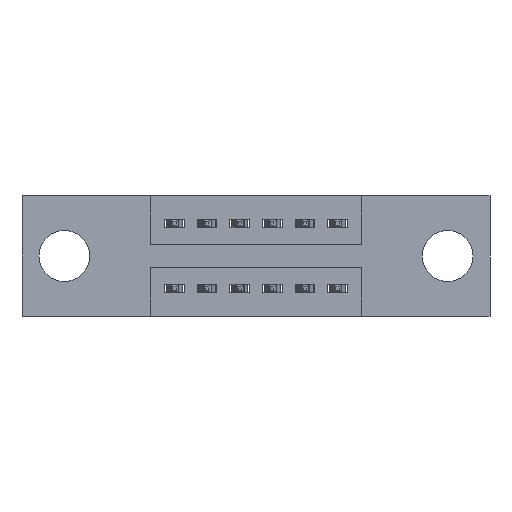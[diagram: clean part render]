
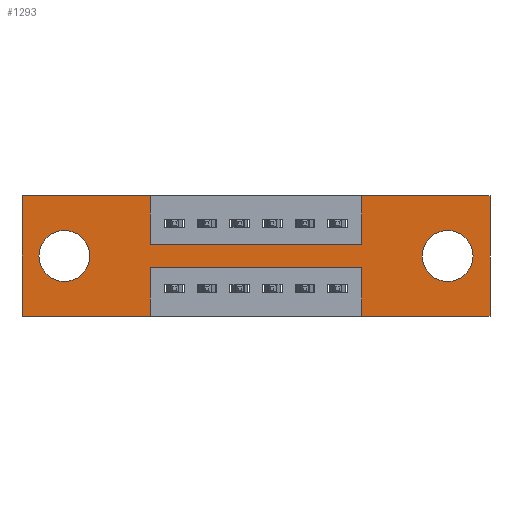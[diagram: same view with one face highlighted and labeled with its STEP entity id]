
A CAD part, front view. The second image highlights one B-rep face of the part: STEP entity #1293.
In plain terms, the highlighted planar face has unit normal (0, -1, 0).
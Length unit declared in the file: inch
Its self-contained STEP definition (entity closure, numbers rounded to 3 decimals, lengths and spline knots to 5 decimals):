
#25 = CIRCLE ( 'NONE', #4524, 0.078 ) ;
#283 = DIRECTION ( 'NONE',  ( 0., 0., -1. ) ) ;
#341 = LINE ( 'NONE', #4122, #7410 ) ;
#418 = ORIENTED_EDGE ( 'NONE', *, *, #1157, .F. ) ;
#460 = DIRECTION ( 'NONE',  ( 0., 0., -1. ) ) ;
#494 = CARTESIAN_POINT ( 'NONE',  ( 1.305, 0., -0.107 ) ) ;
#510 = EDGE_LOOP ( 'NONE', ( #1317, #1648 ) ) ;
#620 = LINE ( 'NONE', #7387, #4422 ) ;
#625 = DIRECTION ( 'NONE',  ( -1., 0., 0. ) ) ;
#694 = VERTEX_POINT ( 'NONE', #2795 ) ;
#718 = VERTEX_POINT ( 'NONE', #4120 ) ;
#769 = CIRCLE ( 'NONE', #6094, 0.078 ) ;
#886 = FACE_BOUND ( 'NONE', #6530, .T. ) ;
#954 = CIRCLE ( 'NONE', #10007, 0.078 ) ;
#986 = FACE_OUTER_BOUND ( 'NONE', #4575, .T. ) ;
#1023 = EDGE_CURVE ( 'NONE', #3708, #5567, #769, .T. ) ;
#1129 = CARTESIAN_POINT ( 'NONE',  ( 1.0425, 0., -0.22 ) ) ;
#1147 = DIRECTION ( 'NONE',  ( -1., 0., 0. ) ) ;
#1157 = EDGE_CURVE ( 'NONE', #1844, #1894, #1882, .T. ) ;
#1201 = ORIENTED_EDGE ( 'NONE', *, *, #7354, .F. ) ;
#1293 = ADVANCED_FACE ( 'NONE', ( #6348, #886, #986 ), #5481, .T. ) ;
#1317 = ORIENTED_EDGE ( 'NONE', *, *, #2758, .T. ) ;
#1533 = LINE ( 'NONE', #6993, #7560 ) ;
#1587 = DIRECTION ( 'NONE',  ( 0., -1., 0. ) ) ;
#1648 = ORIENTED_EDGE ( 'NONE', *, *, #5565, .T. ) ;
#1691 = VECTOR ( 'NONE', #9015, 39.37008 ) ;
#1844 = VERTEX_POINT ( 'NONE', #9425 ) ;
#1871 = VERTEX_POINT ( 'NONE', #9616 ) ;
#1877 = CARTESIAN_POINT ( 'NONE',  ( 1.0425, 0., -0.15 ) ) ;
#1879 = AXIS2_PLACEMENT_3D ( 'NONE', #3194, #1587, #8573 ) ;
#1882 = LINE ( 'NONE', #6601, #3819 ) ;
#1894 = VERTEX_POINT ( 'NONE', #2571 ) ;
#1993 = VERTEX_POINT ( 'NONE', #7368 ) ;
#2045 = VERTEX_POINT ( 'NONE', #494 ) ;
#2224 = VECTOR ( 'NONE', #4708, 39.37008 ) ;
#2343 = EDGE_CURVE ( 'NONE', #6009, #1993, #5828, .T. ) ;
#2400 = DIRECTION ( 'NONE',  ( 0., 1., 0. ) ) ;
#2403 = EDGE_CURVE ( 'NONE', #694, #2716, #3394, .T. ) ;
#2435 = CARTESIAN_POINT ( 'NONE',  ( 1.435, 0., 0. ) ) ;
#2571 = CARTESIAN_POINT ( 'NONE',  ( 0.3925, 0., -0.37 ) ) ;
#2659 = ORIENTED_EDGE ( 'NONE', *, *, #7811, .F. ) ;
#2703 = CARTESIAN_POINT ( 'NONE',  ( 1.435, 0., 0. ) ) ;
#2705 = ORIENTED_EDGE ( 'NONE', *, *, #9363, .F. ) ;
#2716 = VERTEX_POINT ( 'NONE', #1129 ) ;
#2758 = EDGE_CURVE ( 'NONE', #2045, #718, #954, .T. ) ;
#2795 = CARTESIAN_POINT ( 'NONE',  ( 1.0425, 0., -0.37 ) ) ;
#2916 = DIRECTION ( 'NONE',  ( 0., 0., -1. ) ) ;
#3032 = VECTOR ( 'NONE', #9635, 39.37008 ) ;
#3147 = EDGE_CURVE ( 'NONE', #3807, #1871, #9086, .T. ) ;
#3194 = CARTESIAN_POINT ( 'NONE',  ( 0., 0., -0.37 ) ) ;
#3263 = VECTOR ( 'NONE', #6921, 39.37008 ) ;
#3394 = LINE ( 'NONE', #7202, #3032 ) ;
#3422 = VERTEX_POINT ( 'NONE', #2703 ) ;
#3441 = EDGE_CURVE ( 'NONE', #8538, #694, #341, .T. ) ;
#3496 = ORIENTED_EDGE ( 'NONE', *, *, #6193, .F. ) ;
#3680 = VECTOR ( 'NONE', #5234, 39.37008 ) ;
#3708 = VERTEX_POINT ( 'NONE', #4154 ) ;
#3766 = CARTESIAN_POINT ( 'NONE',  ( 1.0425, 0., 0. ) ) ;
#3768 = LINE ( 'NONE', #5288, #3263 ) ;
#3772 = VERTEX_POINT ( 'NONE', #1877 ) ;
#3795 = CARTESIAN_POINT ( 'NONE',  ( 0., 0., -0.37 ) ) ;
#3807 = VERTEX_POINT ( 'NONE', #9681 ) ;
#3819 = VECTOR ( 'NONE', #283, 39.37008 ) ;
#3835 = EDGE_CURVE ( 'NONE', #5567, #3708, #25, .T. ) ;
#3990 = LINE ( 'NONE', #2435, #2224 ) ;
#4120 = CARTESIAN_POINT ( 'NONE',  ( 1.305, 0., -0.263 ) ) ;
#4122 = CARTESIAN_POINT ( 'NONE',  ( 0., 0., -0.37 ) ) ;
#4154 = CARTESIAN_POINT ( 'NONE',  ( 0.13, 0., -0.107 ) ) ;
#4225 = AXIS2_PLACEMENT_3D ( 'NONE', #4339, #8139, #2916 ) ;
#4233 = DIRECTION ( 'NONE',  ( 1., 0., 0. ) ) ;
#4273 = EDGE_CURVE ( 'NONE', #1993, #3772, #5080, .T. ) ;
#4339 = CARTESIAN_POINT ( 'NONE',  ( 1.305, 0., -0.185 ) ) ;
#4422 = VECTOR ( 'NONE', #5146, 39.37008 ) ;
#4524 = AXIS2_PLACEMENT_3D ( 'NONE', #7440, #9062, #5823 ) ;
#4575 = EDGE_LOOP ( 'NONE', ( #418, #2659, #7725, #9198, #2705, #4729, #1201, #6831, #7426, #3496, #5720, #9352 ) ) ;
#4708 = DIRECTION ( 'NONE',  ( 0., 0., -1. ) ) ;
#4729 = ORIENTED_EDGE ( 'NONE', *, *, #9469, .F. ) ;
#4903 = VERTEX_POINT ( 'NONE', #3766 ) ;
#5080 = LINE ( 'NONE', #5136, #6509 ) ;
#5136 = CARTESIAN_POINT ( 'NONE',  ( 0.3925, 0., -0.15 ) ) ;
#5146 = DIRECTION ( 'NONE',  ( -1., 0., 0. ) ) ;
#5150 = LINE ( 'NONE', #3795, #9935 ) ;
#5234 = DIRECTION ( 'NONE',  ( 0., 0., 1. ) ) ;
#5288 = CARTESIAN_POINT ( 'NONE',  ( 0., 0., 0. ) ) ;
#5475 = DIRECTION ( 'NONE',  ( 1., 0., 0. ) ) ;
#5481 = PLANE ( 'NONE',  #1879 ) ;
#5492 = DIRECTION ( 'NONE',  ( 0., 0., 1. ) ) ;
#5565 = EDGE_CURVE ( 'NONE', #718, #2045, #6992, .T. ) ;
#5567 = VERTEX_POINT ( 'NONE', #7430 ) ;
#5720 = ORIENTED_EDGE ( 'NONE', *, *, #3147, .F. ) ;
#5785 = CARTESIAN_POINT ( 'NONE',  ( 0.3925, 0., 0. ) ) ;
#5823 = DIRECTION ( 'NONE',  ( 0., 0., 1. ) ) ;
#5828 = LINE ( 'NONE', #5785, #5926 ) ;
#5926 = VECTOR ( 'NONE', #9732, 39.37008 ) ;
#6009 = VERTEX_POINT ( 'NONE', #8890 ) ;
#6094 = AXIS2_PLACEMENT_3D ( 'NONE', #7013, #2400, #5492 ) ;
#6168 = CARTESIAN_POINT ( 'NONE',  ( 0., 0., 0. ) ) ;
#6193 = EDGE_CURVE ( 'NONE', #1871, #6009, #3768, .T. ) ;
#6348 = FACE_BOUND ( 'NONE', #510, .T. ) ;
#6492 = CARTESIAN_POINT ( 'NONE',  ( 1.305, 0., -0.185 ) ) ;
#6509 = VECTOR ( 'NONE', #4233, 39.37008 ) ;
#6530 = EDGE_LOOP ( 'NONE', ( #7527, #9460 ) ) ;
#6601 = CARTESIAN_POINT ( 'NONE',  ( 0.3925, 0., -0.37 ) ) ;
#6831 = ORIENTED_EDGE ( 'NONE', *, *, #4273, .F. ) ;
#6921 = DIRECTION ( 'NONE',  ( 1., 0., 0. ) ) ;
#6992 = CIRCLE ( 'NONE', #4225, 0.078 ) ;
#6993 = CARTESIAN_POINT ( 'NONE',  ( 0., 0., 0. ) ) ;
#7013 = CARTESIAN_POINT ( 'NONE',  ( 0.13, 0., -0.185 ) ) ;
#7109 = EDGE_CURVE ( 'NONE', #1894, #3807, #5150, .T. ) ;
#7202 = CARTESIAN_POINT ( 'NONE',  ( 1.0425, 0., -0.37 ) ) ;
#7354 = EDGE_CURVE ( 'NONE', #3772, #4903, #9894, .T. ) ;
#7368 = CARTESIAN_POINT ( 'NONE',  ( 0.3925, 0., -0.15 ) ) ;
#7384 = DIRECTION ( 'NONE',  ( 0., 1., 0. ) ) ;
#7387 = CARTESIAN_POINT ( 'NONE',  ( 0.3925, 0., -0.22 ) ) ;
#7410 = VECTOR ( 'NONE', #1147, 39.37008 ) ;
#7426 = ORIENTED_EDGE ( 'NONE', *, *, #2343, .F. ) ;
#7430 = CARTESIAN_POINT ( 'NONE',  ( 0.13, 0., -0.263 ) ) ;
#7440 = CARTESIAN_POINT ( 'NONE',  ( 0.13, 0., -0.185 ) ) ;
#7527 = ORIENTED_EDGE ( 'NONE', *, *, #1023, .T. ) ;
#7560 = VECTOR ( 'NONE', #5475, 39.37008 ) ;
#7637 = CARTESIAN_POINT ( 'NONE',  ( 1.435, 0., -0.37 ) ) ;
#7725 = ORIENTED_EDGE ( 'NONE', *, *, #2403, .F. ) ;
#7811 = EDGE_CURVE ( 'NONE', #2716, #1844, #620, .T. ) ;
#8139 = DIRECTION ( 'NONE',  ( 0., 1., 0. ) ) ;
#8538 = VERTEX_POINT ( 'NONE', #7637 ) ;
#8573 = DIRECTION ( 'NONE',  ( 0., 0., -1. ) ) ;
#8890 = CARTESIAN_POINT ( 'NONE',  ( 0.3925, 0., 0. ) ) ;
#9015 = DIRECTION ( 'NONE',  ( 0., 0., 1. ) ) ;
#9062 = DIRECTION ( 'NONE',  ( 0., 1., 0. ) ) ;
#9086 = LINE ( 'NONE', #6168, #3680 ) ;
#9198 = ORIENTED_EDGE ( 'NONE', *, *, #3441, .F. ) ;
#9352 = ORIENTED_EDGE ( 'NONE', *, *, #7109, .F. ) ;
#9363 = EDGE_CURVE ( 'NONE', #3422, #8538, #3990, .T. ) ;
#9425 = CARTESIAN_POINT ( 'NONE',  ( 0.3925, 0., -0.22 ) ) ;
#9460 = ORIENTED_EDGE ( 'NONE', *, *, #3835, .T. ) ;
#9469 = EDGE_CURVE ( 'NONE', #4903, #3422, #1533, .T. ) ;
#9616 = CARTESIAN_POINT ( 'NONE',  ( 0., 0., 0. ) ) ;
#9635 = DIRECTION ( 'NONE',  ( 0., 0., 1. ) ) ;
#9681 = CARTESIAN_POINT ( 'NONE',  ( 0., 0., -0.37 ) ) ;
#9732 = DIRECTION ( 'NONE',  ( 0., 0., -1. ) ) ;
#9894 = LINE ( 'NONE', #9949, #1691 ) ;
#9935 = VECTOR ( 'NONE', #625, 39.37008 ) ;
#9949 = CARTESIAN_POINT ( 'NONE',  ( 1.0425, 0., 0. ) ) ;
#10007 = AXIS2_PLACEMENT_3D ( 'NONE', #6492, #7384, #460 ) ;
